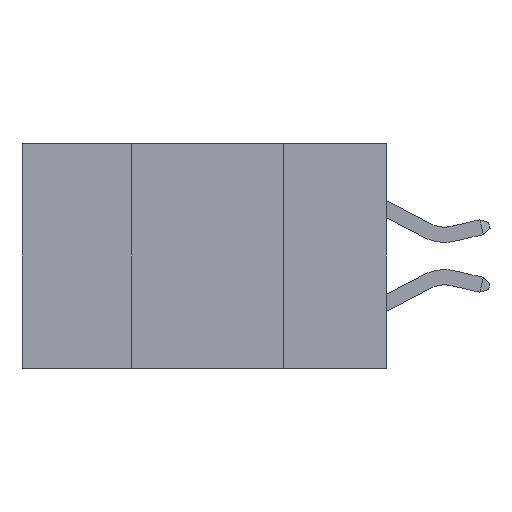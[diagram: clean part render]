
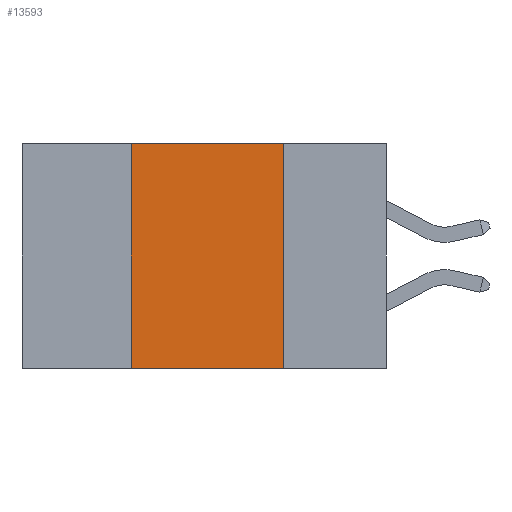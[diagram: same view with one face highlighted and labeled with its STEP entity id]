
A CAD part, left-side view. The second image highlights one B-rep face of the part: STEP entity #13593.
In plain terms, the highlighted planar face has unit normal (-1, 0, 0).
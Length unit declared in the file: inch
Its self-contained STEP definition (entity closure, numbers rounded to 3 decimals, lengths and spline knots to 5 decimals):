
#295 = VERTEX_POINT ( 'NONE', #7447 ) ;
#1785 = EDGE_CURVE ( 'NONE', #1942, #12477, #5613, .T. ) ;
#1942 = VERTEX_POINT ( 'NONE', #4751 ) ;
#2649 = VECTOR ( 'NONE', #9918, 39.37008 ) ;
#3559 = EDGE_LOOP ( 'NONE', ( #9646, #6252, #6174, #9757 ) ) ;
#3969 = FACE_OUTER_BOUND ( 'NONE', #3559, .T. ) ;
#4751 = CARTESIAN_POINT ( 'NONE',  ( 0., 0.42, 0. ) ) ;
#4981 = CARTESIAN_POINT ( 'NONE',  ( 0., 0.6, 0. ) ) ;
#5613 = LINE ( 'NONE', #13504, #10127 ) ;
#5880 = CARTESIAN_POINT ( 'NONE',  ( 0., 0.42, -0.37 ) ) ;
#6174 = ORIENTED_EDGE ( 'NONE', *, *, #11056, .F. ) ;
#6252 = ORIENTED_EDGE ( 'NONE', *, *, #1785, .F. ) ;
#6309 = DIRECTION ( 'NONE',  ( 1., 0., 0. ) ) ;
#6359 = CARTESIAN_POINT ( 'NONE',  ( 0., 0.17, -0.37 ) ) ;
#6993 = VECTOR ( 'NONE', #11581, 39.37008 ) ;
#7447 = CARTESIAN_POINT ( 'NONE',  ( 0., 0.42, -0.37 ) ) ;
#8627 = AXIS2_PLACEMENT_3D ( 'NONE', #4981, #6309, #8862 ) ;
#8862 = DIRECTION ( 'NONE',  ( 0., 0., -1. ) ) ;
#8911 = LINE ( 'NONE', #12874, #6993 ) ;
#9646 = ORIENTED_EDGE ( 'NONE', *, *, #10821, .F. ) ;
#9655 = LINE ( 'NONE', #16183, #2649 ) ;
#9757 = ORIENTED_EDGE ( 'NONE', *, *, #15437, .T. ) ;
#9836 = VERTEX_POINT ( 'NONE', #6359 ) ;
#9918 = DIRECTION ( 'NONE',  ( 0., 0., -1. ) ) ;
#10127 = VECTOR ( 'NONE', #10882, 39.37008 ) ;
#10545 = CARTESIAN_POINT ( 'NONE',  ( 0., 0.17, 0. ) ) ;
#10821 = EDGE_CURVE ( 'NONE', #12477, #9836, #9655, .T. ) ;
#10882 = DIRECTION ( 'NONE',  ( 0., -1., 0. ) ) ;
#11056 = EDGE_CURVE ( 'NONE', #295, #1942, #14826, .T. ) ;
#11581 = DIRECTION ( 'NONE',  ( 0., -1., 0. ) ) ;
#11684 = PLANE ( 'NONE',  #8627 ) ;
#12010 = VECTOR ( 'NONE', #13727, 39.37008 ) ;
#12477 = VERTEX_POINT ( 'NONE', #10545 ) ;
#12874 = CARTESIAN_POINT ( 'NONE',  ( 0., 0.6, -0.37 ) ) ;
#13504 = CARTESIAN_POINT ( 'NONE',  ( 0., 0.6, 0. ) ) ;
#13593 = ADVANCED_FACE ( 'NONE', ( #3969 ), #11684, .F. ) ;
#13727 = DIRECTION ( 'NONE',  ( 0., 0., 1. ) ) ;
#14826 = LINE ( 'NONE', #5880, #12010 ) ;
#15437 = EDGE_CURVE ( 'NONE', #295, #9836, #8911, .T. ) ;
#16183 = CARTESIAN_POINT ( 'NONE',  ( 0., 0.17, -0.37 ) ) ;
